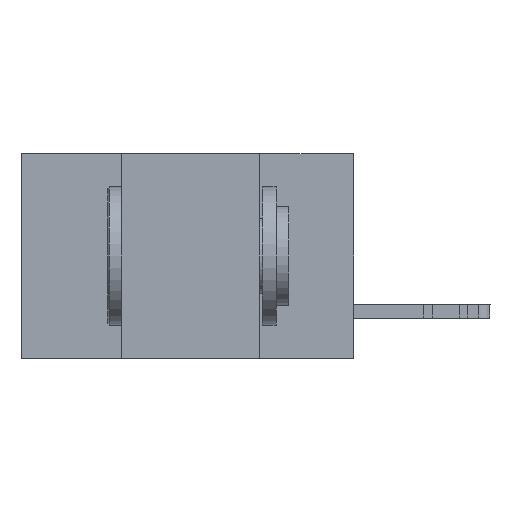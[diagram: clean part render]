
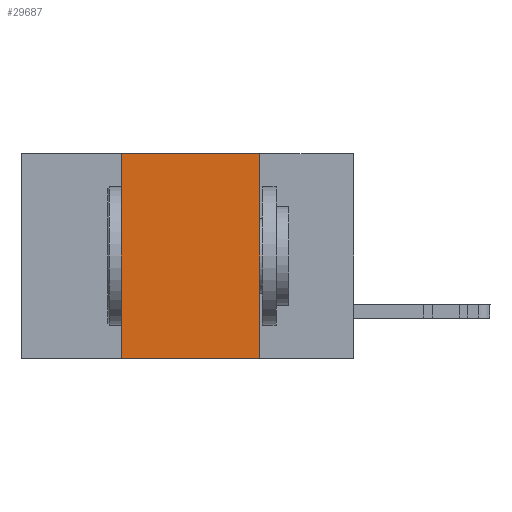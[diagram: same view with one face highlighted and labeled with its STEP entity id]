
A CAD part, left-side view. The second image highlights one B-rep face of the part: STEP entity #29687.
In plain terms, the highlighted planar face has unit normal (-1, 0, 0).
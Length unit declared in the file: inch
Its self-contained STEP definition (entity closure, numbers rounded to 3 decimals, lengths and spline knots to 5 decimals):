
#609 = CARTESIAN_POINT ( 'NONE',  ( 0., 0.42, -0.37 ) ) ;
#838 = LINE ( 'NONE', #18496, #30146 ) ;
#1256 = VERTEX_POINT ( 'NONE', #46355 ) ;
#1560 = ORIENTED_EDGE ( 'NONE', *, *, #4621, .F. ) ;
#3219 = CARTESIAN_POINT ( 'NONE',  ( 0., 0.6, -0.37 ) ) ;
#3551 = VERTEX_POINT ( 'NONE', #609 ) ;
#3808 = CARTESIAN_POINT ( 'NONE',  ( 0., 0.6, 0. ) ) ;
#4621 = EDGE_CURVE ( 'NONE', #38512, #1256, #838, .T. ) ;
#5739 = VECTOR ( 'NONE', #43157, 39.37008 ) ;
#7612 = AXIS2_PLACEMENT_3D ( 'NONE', #3808, #40776, #43645 ) ;
#7856 = PLANE ( 'NONE',  #7612 ) ;
#12111 = EDGE_LOOP ( 'NONE', ( #32077, #1560, #22495, #32632 ) ) ;
#18496 = CARTESIAN_POINT ( 'NONE',  ( 0., 0.6, 0. ) ) ;
#19014 = VERTEX_POINT ( 'NONE', #31406 ) ;
#22087 = CARTESIAN_POINT ( 'NONE',  ( 0., 0.42, 0. ) ) ;
#22495 = ORIENTED_EDGE ( 'NONE', *, *, #45329, .F. ) ;
#25410 = EDGE_CURVE ( 'NONE', #1256, #19014, #46721, .T. ) ;
#28216 = VECTOR ( 'NONE', #46170, 39.37008 ) ;
#28288 = LINE ( 'NONE', #3219, #28216 ) ;
#28601 = CARTESIAN_POINT ( 'NONE',  ( 0., 0.17, 0. ) ) ;
#29687 = ADVANCED_FACE ( 'NONE', ( #32681 ), #7856, .F. ) ;
#30146 = VECTOR ( 'NONE', #33048, 39.37008 ) ;
#30516 = EDGE_CURVE ( 'NONE', #3551, #19014, #28288, .T. ) ;
#31406 = CARTESIAN_POINT ( 'NONE',  ( 0., 0.17, -0.37 ) ) ;
#32077 = ORIENTED_EDGE ( 'NONE', *, *, #25410, .F. ) ;
#32632 = ORIENTED_EDGE ( 'NONE', *, *, #30516, .T. ) ;
#32681 = FACE_OUTER_BOUND ( 'NONE', #12111, .T. ) ;
#33048 = DIRECTION ( 'NONE',  ( 0., -1., 0. ) ) ;
#33871 = CARTESIAN_POINT ( 'NONE',  ( 0., 0.42, 0. ) ) ;
#38512 = VERTEX_POINT ( 'NONE', #33871 ) ;
#40671 = DIRECTION ( 'NONE',  ( 0., 0., 1. ) ) ;
#40776 = DIRECTION ( 'NONE',  ( 1., 0., 0. ) ) ;
#43157 = DIRECTION ( 'NONE',  ( 0., 0., -1. ) ) ;
#43321 = LINE ( 'NONE', #22087, #43882 ) ;
#43645 = DIRECTION ( 'NONE',  ( 0., 0., -1. ) ) ;
#43882 = VECTOR ( 'NONE', #40671, 39.37008 ) ;
#45329 = EDGE_CURVE ( 'NONE', #3551, #38512, #43321, .T. ) ;
#46170 = DIRECTION ( 'NONE',  ( 0., -1., 0. ) ) ;
#46355 = CARTESIAN_POINT ( 'NONE',  ( 0., 0.17, 0. ) ) ;
#46721 = LINE ( 'NONE', #28601, #5739 ) ;
